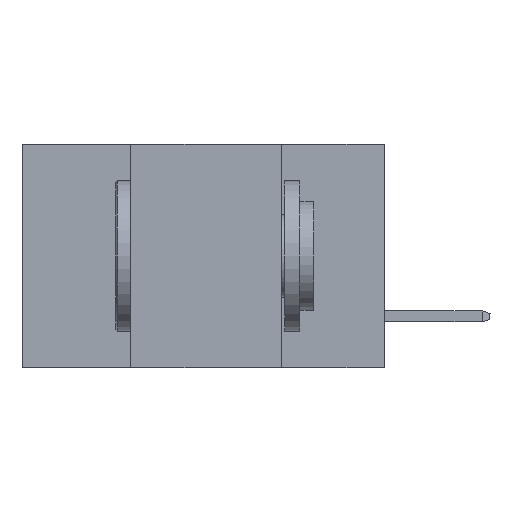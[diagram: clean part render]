
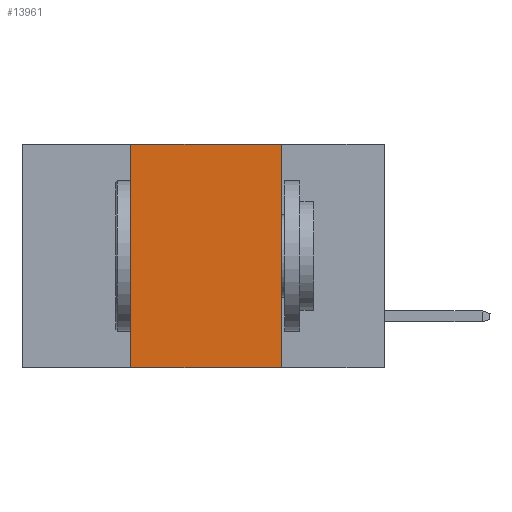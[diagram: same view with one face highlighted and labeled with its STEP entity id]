
A CAD part, left-side view. The second image highlights one B-rep face of the part: STEP entity #13961.
In plain terms, the highlighted planar face has unit normal (-1, 0, 0).
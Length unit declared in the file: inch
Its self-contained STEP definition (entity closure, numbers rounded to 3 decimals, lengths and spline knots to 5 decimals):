
#340 = DIRECTION ( 'NONE',  ( 0., 0., -1. ) ) ;
#581 = CARTESIAN_POINT ( 'NONE',  ( 0., 0.6, 0. ) ) ;
#2174 = EDGE_LOOP ( 'NONE', ( #9730, #16475, #16282, #11242 ) ) ;
#3448 = VECTOR ( 'NONE', #5920, 39.37008 ) ;
#3450 = VECTOR ( 'NONE', #19757, 39.37008 ) ;
#4465 = LINE ( 'NONE', #17416, #9828 ) ;
#5022 = EDGE_CURVE ( 'NONE', #16217, #11008, #16739, .T. ) ;
#5725 = AXIS2_PLACEMENT_3D ( 'NONE', #581, #8209, #17785 ) ;
#5920 = DIRECTION ( 'NONE',  ( 0., -1., 0. ) ) ;
#6714 = VERTEX_POINT ( 'NONE', #13376 ) ;
#7681 = VERTEX_POINT ( 'NONE', #23221 ) ;
#8209 = DIRECTION ( 'NONE',  ( 1., 0., 0. ) ) ;
#9730 = ORIENTED_EDGE ( 'NONE', *, *, #19366, .F. ) ;
#9801 = DIRECTION ( 'NONE',  ( 0., 0., 1. ) ) ;
#9828 = VECTOR ( 'NONE', #340, 39.37008 ) ;
#11008 = VERTEX_POINT ( 'NONE', #19802 ) ;
#11242 = ORIENTED_EDGE ( 'NONE', *, *, #5022, .T. ) ;
#12038 = CARTESIAN_POINT ( 'NONE',  ( 0., 0.42, -0.37 ) ) ;
#13029 = CARTESIAN_POINT ( 'NONE',  ( 0., 0.6, -0.37 ) ) ;
#13376 = CARTESIAN_POINT ( 'NONE',  ( 0., 0.42, 0. ) ) ;
#13427 = VECTOR ( 'NONE', #9801, 39.37008 ) ;
#13900 = LINE ( 'NONE', #12038, #13427 ) ;
#13937 = CARTESIAN_POINT ( 'NONE',  ( 0., 0.6, 0. ) ) ;
#13961 = ADVANCED_FACE ( 'NONE', ( #14309 ), #21873, .F. ) ;
#14309 = FACE_OUTER_BOUND ( 'NONE', #2174, .T. ) ;
#15795 = LINE ( 'NONE', #13937, #3450 ) ;
#16217 = VERTEX_POINT ( 'NONE', #22929 ) ;
#16282 = ORIENTED_EDGE ( 'NONE', *, *, #18466, .F. ) ;
#16475 = ORIENTED_EDGE ( 'NONE', *, *, #19343, .F. ) ;
#16739 = LINE ( 'NONE', #13029, #3448 ) ;
#17416 = CARTESIAN_POINT ( 'NONE',  ( 0., 0.17, -0.37 ) ) ;
#17785 = DIRECTION ( 'NONE',  ( 0., 0., -1. ) ) ;
#18466 = EDGE_CURVE ( 'NONE', #16217, #6714, #13900, .T. ) ;
#19343 = EDGE_CURVE ( 'NONE', #6714, #7681, #15795, .T. ) ;
#19366 = EDGE_CURVE ( 'NONE', #7681, #11008, #4465, .T. ) ;
#19757 = DIRECTION ( 'NONE',  ( 0., -1., 0. ) ) ;
#19802 = CARTESIAN_POINT ( 'NONE',  ( 0., 0.17, -0.37 ) ) ;
#21873 = PLANE ( 'NONE',  #5725 ) ;
#22929 = CARTESIAN_POINT ( 'NONE',  ( 0., 0.42, -0.37 ) ) ;
#23221 = CARTESIAN_POINT ( 'NONE',  ( 0., 0.17, 0. ) ) ;
